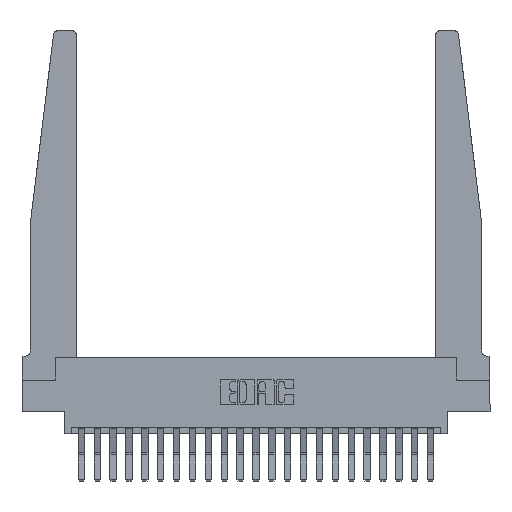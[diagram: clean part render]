
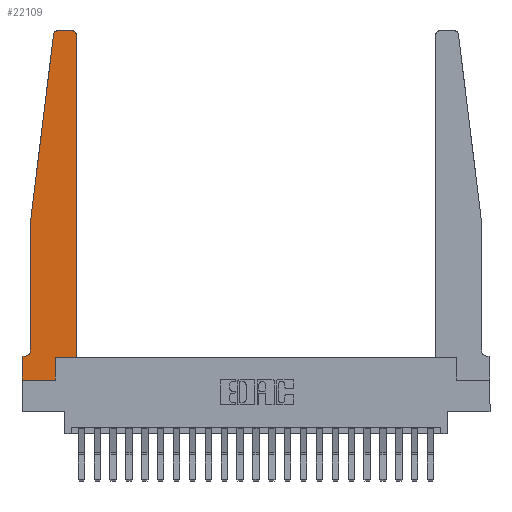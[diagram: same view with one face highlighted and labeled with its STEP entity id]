
A CAD part, top view. The second image highlights one B-rep face of the part: STEP entity #22109.
In plain terms, the highlighted planar face has unit normal (0, 0, 1).
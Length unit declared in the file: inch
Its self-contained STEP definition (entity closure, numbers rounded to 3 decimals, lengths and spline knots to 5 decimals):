
#154 = CARTESIAN_POINT ( 'NONE',  ( 0.015, 0.1875, 0.37 ) ) ;
#160 = VERTEX_POINT ( 'NONE', #18892 ) ;
#339 = VERTEX_POINT ( 'NONE', #154 ) ;
#557 = CARTESIAN_POINT ( 'NONE',  ( 0.24675, 2.72367, 0.37 ) ) ;
#734 = ORIENTED_EDGE ( 'NONE', *, *, #20351, .T. ) ;
#915 = ORIENTED_EDGE ( 'NONE', *, *, #11276, .T. ) ;
#924 = CARTESIAN_POINT ( 'NONE',  ( 0.425, 2.72, 0.37 ) ) ;
#1010 = LINE ( 'NONE', #8092, #17422 ) ;
#1267 = VERTEX_POINT ( 'NONE', #557 ) ;
#1312 = ORIENTED_EDGE ( 'NONE', *, *, #12646, .T. ) ;
#1808 = EDGE_LOOP ( 'NONE', ( #734, #10277, #2530, #14021, #3980, #22604, #16751, #6070, #1312, #915, #12416, #7832 ) ) ;
#1855 = CARTESIAN_POINT ( 'NONE',  ( 0.065, 1.25, 0.37 ) ) ;
#2224 = CIRCLE ( 'NONE', #2962, 0.05 ) ;
#2530 = ORIENTED_EDGE ( 'NONE', *, *, #8338, .T. ) ;
#2579 = EDGE_CURVE ( 'NONE', #160, #10768, #21299, .T. ) ;
#2962 = AXIS2_PLACEMENT_3D ( 'NONE', #9484, #7408, #19776 ) ;
#3006 = VECTOR ( 'NONE', #6954, 39.37008 ) ;
#3168 = VECTOR ( 'NONE', #13022, 39.37008 ) ;
#3482 = CARTESIAN_POINT ( 'NONE',  ( 0.27653, 2.75, 0.37 ) ) ;
#3524 = CIRCLE ( 'NONE', #18452, 0.03 ) ;
#3852 = CARTESIAN_POINT ( 'NONE',  ( 0.425, 0.18, 0.37 ) ) ;
#3965 = DIRECTION ( 'NONE',  ( 0., 0., 1. ) ) ;
#3980 = ORIENTED_EDGE ( 'NONE', *, *, #8847, .T. ) ;
#4029 = DIRECTION ( 'NONE',  ( 0., 0., 1. ) ) ;
#4504 = CARTESIAN_POINT ( 'NONE',  ( 0.065, 0.1875, 0.37 ) ) ;
#4790 = VECTOR ( 'NONE', #21078, 39.37008 ) ;
#4900 = VECTOR ( 'NONE', #22698, 39.37008 ) ;
#5293 = CARTESIAN_POINT ( 'NONE',  ( 0.2605, 0., 0.37 ) ) ;
#5888 = DIRECTION ( 'NONE',  ( 1., 0., 0. ) ) ;
#6070 = ORIENTED_EDGE ( 'NONE', *, *, #22132, .T. ) ;
#6257 = VERTEX_POINT ( 'NONE', #22284 ) ;
#6359 = CARTESIAN_POINT ( 'NONE',  ( 0.2605, 0.18, 0.37 ) ) ;
#6387 = LINE ( 'NONE', #18855, #4900 ) ;
#6859 = VECTOR ( 'NONE', #11931, 39.37008 ) ;
#6863 = LINE ( 'NONE', #19336, #7869 ) ;
#6954 = DIRECTION ( 'NONE',  ( 0., -1., 0. ) ) ;
#7373 = VERTEX_POINT ( 'NONE', #5293 ) ;
#7395 = DIRECTION ( 'NONE',  ( 1., 0., 0. ) ) ;
#7408 = DIRECTION ( 'NONE',  ( 0., 0., -1. ) ) ;
#7536 = CARTESIAN_POINT ( 'NONE',  ( 0., 0., 0.37 ) ) ;
#7537 = CARTESIAN_POINT ( 'NONE',  ( 0.395, 2.75, 0.37 ) ) ;
#7832 = ORIENTED_EDGE ( 'NONE', *, *, #13300, .T. ) ;
#7869 = VECTOR ( 'NONE', #15721, 39.37008 ) ;
#7963 = LINE ( 'NONE', #14853, #10505 ) ;
#8092 = CARTESIAN_POINT ( 'NONE',  ( 0.425, 0.18, 0.37 ) ) ;
#8338 = EDGE_CURVE ( 'NONE', #1267, #160, #14090, .T. ) ;
#8351 = LINE ( 'NONE', #20833, #19276 ) ;
#8847 = EDGE_CURVE ( 'NONE', #10768, #339, #2224, .T. ) ;
#9066 = DIRECTION ( 'NONE',  ( 1., 0., 0. ) ) ;
#9484 = CARTESIAN_POINT ( 'NONE',  ( 0.015, 0.2375, 0.37 ) ) ;
#9592 = DIRECTION ( 'NONE',  ( 0., 0., 1. ) ) ;
#9610 = LINE ( 'NONE', #18260, #3168 ) ;
#10277 = ORIENTED_EDGE ( 'NONE', *, *, #21668, .T. ) ;
#10505 = VECTOR ( 'NONE', #16361, 39.37008 ) ;
#10768 = VERTEX_POINT ( 'NONE', #12736 ) ;
#11262 = VERTEX_POINT ( 'NONE', #924 ) ;
#11276 = EDGE_CURVE ( 'NONE', #19511, #16484, #6387, .T. ) ;
#11931 = DIRECTION ( 'NONE',  ( -1., 0., 0. ) ) ;
#11969 = DIRECTION ( 'NONE',  ( 0., 1., 0. ) ) ;
#12413 = FACE_OUTER_BOUND ( 'NONE', #1808, .T. ) ;
#12416 = ORIENTED_EDGE ( 'NONE', *, *, #18148, .T. ) ;
#12646 = EDGE_CURVE ( 'NONE', #7373, #19511, #8351, .T. ) ;
#12736 = CARTESIAN_POINT ( 'NONE',  ( 0.065, 0.2375, 0.37 ) ) ;
#12914 = VERTEX_POINT ( 'NONE', #7536 ) ;
#13004 = CARTESIAN_POINT ( 'NONE',  ( 0.395, 2.72, 0.37 ) ) ;
#13022 = DIRECTION ( 'NONE',  ( 0., -1., 0. ) ) ;
#13243 = LINE ( 'NONE', #4504, #6859 ) ;
#13300 = EDGE_CURVE ( 'NONE', #11262, #17040, #3524, .T. ) ;
#13848 = EDGE_CURVE ( 'NONE', #6257, #12914, #9610, .T. ) ;
#13955 = EDGE_CURVE ( 'NONE', #339, #6257, #13243, .T. ) ;
#14021 = ORIENTED_EDGE ( 'NONE', *, *, #2579, .T. ) ;
#14090 = LINE ( 'NONE', #21191, #4790 ) ;
#14283 = CARTESIAN_POINT ( 'NONE',  ( 0., 0.1875, 0.37 ) ) ;
#14853 = CARTESIAN_POINT ( 'NONE',  ( 0., 0., 0.37 ) ) ;
#15717 = CIRCLE ( 'NONE', #22048, 0.03 ) ;
#15721 = DIRECTION ( 'NONE',  ( -1., 0., 0. ) ) ;
#16361 = DIRECTION ( 'NONE',  ( 1., 0., 0. ) ) ;
#16484 = VERTEX_POINT ( 'NONE', #3852 ) ;
#16717 = VERTEX_POINT ( 'NONE', #3482 ) ;
#16751 = ORIENTED_EDGE ( 'NONE', *, *, #13848, .T. ) ;
#17040 = VERTEX_POINT ( 'NONE', #7537 ) ;
#17422 = VECTOR ( 'NONE', #20342, 39.37008 ) ;
#18148 = EDGE_CURVE ( 'NONE', #16484, #11262, #1010, .T. ) ;
#18260 = CARTESIAN_POINT ( 'NONE',  ( 0., 0., 0.37 ) ) ;
#18452 = AXIS2_PLACEMENT_3D ( 'NONE', #13004, #4029, #7395 ) ;
#18728 = AXIS2_PLACEMENT_3D ( 'NONE', #14283, #9592, #5888 ) ;
#18855 = CARTESIAN_POINT ( 'NONE',  ( 0.425, 0.18, 0.37 ) ) ;
#18892 = CARTESIAN_POINT ( 'NONE',  ( 0.065, 1.25, 0.37 ) ) ;
#19276 = VECTOR ( 'NONE', #11969, 39.37008 ) ;
#19336 = CARTESIAN_POINT ( 'NONE',  ( 0.25, 2.75, 0.37 ) ) ;
#19511 = VERTEX_POINT ( 'NONE', #6359 ) ;
#19523 = PLANE ( 'NONE',  #18728 ) ;
#19776 = DIRECTION ( 'NONE',  ( -1., 0., 0. ) ) ;
#20342 = DIRECTION ( 'NONE',  ( 0., 1., 0. ) ) ;
#20351 = EDGE_CURVE ( 'NONE', #17040, #16717, #6863, .T. ) ;
#20833 = CARTESIAN_POINT ( 'NONE',  ( 0.2605, 0.18, 0.37 ) ) ;
#21078 = DIRECTION ( 'NONE',  ( -0.122, -0.992, 0. ) ) ;
#21191 = CARTESIAN_POINT ( 'NONE',  ( 0.065, 1.25, 0.37 ) ) ;
#21299 = LINE ( 'NONE', #1855, #3006 ) ;
#21668 = EDGE_CURVE ( 'NONE', #16717, #1267, #15717, .T. ) ;
#22048 = AXIS2_PLACEMENT_3D ( 'NONE', #22844, #3965, #9066 ) ;
#22109 = ADVANCED_FACE ( 'NONE', ( #12413 ), #19523, .T. ) ;
#22132 = EDGE_CURVE ( 'NONE', #12914, #7373, #7963, .T. ) ;
#22284 = CARTESIAN_POINT ( 'NONE',  ( 0., 0.1875, 0.37 ) ) ;
#22604 = ORIENTED_EDGE ( 'NONE', *, *, #13955, .T. ) ;
#22698 = DIRECTION ( 'NONE',  ( 1., 0., 0. ) ) ;
#22844 = CARTESIAN_POINT ( 'NONE',  ( 0.27653, 2.72, 0.37 ) ) ;
